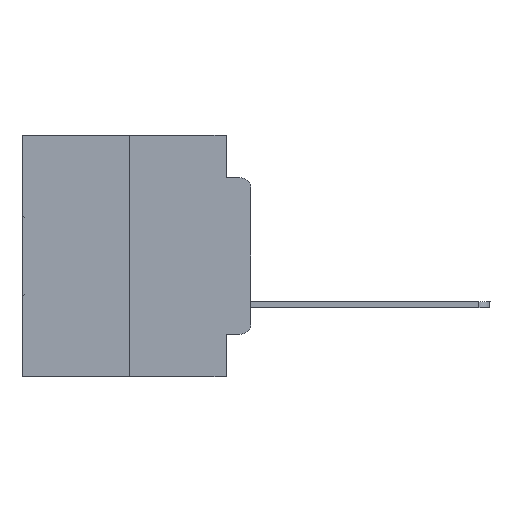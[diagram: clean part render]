
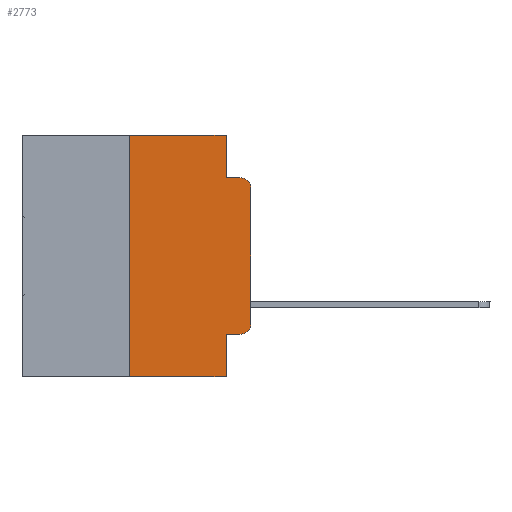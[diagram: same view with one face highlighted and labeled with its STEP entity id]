
A CAD part, left-side view. The second image highlights one B-rep face of the part: STEP entity #2773.
In plain terms, the highlighted planar face has unit normal (-1, 0, 0).
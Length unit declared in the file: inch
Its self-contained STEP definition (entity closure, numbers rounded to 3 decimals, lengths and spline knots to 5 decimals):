
#4 = VERTEX_POINT ( 'NONE', #14316 ) ;
#375 = LINE ( 'NONE', #21339, #31146 ) ;
#378 = CARTESIAN_POINT ( 'NONE',  ( 0., 0.02, -0.0885 ) ) ;
#1081 = VERTEX_POINT ( 'NONE', #2735 ) ;
#2509 = CARTESIAN_POINT ( 'NONE',  ( 0., 0.02, -0.4115 ) ) ;
#2677 = VERTEX_POINT ( 'NONE', #24000 ) ;
#2735 = CARTESIAN_POINT ( 'NONE',  ( 0., 0.051, 0. ) ) ;
#2773 = ADVANCED_FACE ( 'NONE', ( #18692 ), #16845, .F. ) ;
#2887 = CARTESIAN_POINT ( 'NONE',  ( 0., 0., 0. ) ) ;
#3258 = VERTEX_POINT ( 'NONE', #2509 ) ;
#3764 = VECTOR ( 'NONE', #27552, 39.37008 ) ;
#3989 = DIRECTION ( 'NONE',  ( 0., 0., -1. ) ) ;
#4099 = ORIENTED_EDGE ( 'NONE', *, *, #5111, .F. ) ;
#4485 = CARTESIAN_POINT ( 'NONE',  ( 0., 0.051, -0.4115 ) ) ;
#4489 = CARTESIAN_POINT ( 'NONE',  ( 0., 0.051, -0.0885 ) ) ;
#4535 = VERTEX_POINT ( 'NONE', #17187 ) ;
#5091 = CARTESIAN_POINT ( 'NONE',  ( 0., 0.25, 0. ) ) ;
#5111 = EDGE_CURVE ( 'NONE', #12647, #26670, #29083, .T. ) ;
#6140 = CIRCLE ( 'NONE', #15442, 0.02 ) ;
#6686 = CARTESIAN_POINT ( 'NONE',  ( 0., 0.473, -0.5 ) ) ;
#6789 = DIRECTION ( 'NONE',  ( 1., 0., 0. ) ) ;
#6993 = LINE ( 'NONE', #21901, #21143 ) ;
#7224 = VECTOR ( 'NONE', #22726, 39.37008 ) ;
#7760 = ORIENTED_EDGE ( 'NONE', *, *, #19105, .F. ) ;
#8039 = EDGE_CURVE ( 'NONE', #4535, #29188, #31337, .T. ) ;
#8540 = DIRECTION ( 'NONE',  ( 0., -1., 0. ) ) ;
#9163 = DIRECTION ( 'NONE',  ( 0., 0., -1. ) ) ;
#9197 = CARTESIAN_POINT ( 'NONE',  ( 0., 0.02, -0.3915 ) ) ;
#10219 = ORIENTED_EDGE ( 'NONE', *, *, #20925, .T. ) ;
#12647 = VERTEX_POINT ( 'NONE', #20083 ) ;
#12903 = ORIENTED_EDGE ( 'NONE', *, *, #32550, .F. ) ;
#13345 = CARTESIAN_POINT ( 'NONE',  ( 0., 0.051, 0. ) ) ;
#14316 = CARTESIAN_POINT ( 'NONE',  ( 0., 0.051, -0.4115 ) ) ;
#15442 = AXIS2_PLACEMENT_3D ( 'NONE', #9197, #19457, #3989 ) ;
#16789 = ORIENTED_EDGE ( 'NONE', *, *, #24259, .T. ) ;
#16845 = PLANE ( 'NONE',  #33060 ) ;
#16944 = DIRECTION ( 'NONE',  ( 0., 0., -1. ) ) ;
#17187 = CARTESIAN_POINT ( 'NONE',  ( 0., 0.25, -0.5 ) ) ;
#17409 = ORIENTED_EDGE ( 'NONE', *, *, #23856, .T. ) ;
#18180 = EDGE_CURVE ( 'NONE', #4535, #2677, #31624, .T. ) ;
#18672 = LINE ( 'NONE', #13345, #25993 ) ;
#18692 = FACE_OUTER_BOUND ( 'NONE', #29933, .T. ) ;
#19105 = EDGE_CURVE ( 'NONE', #29188, #1081, #375, .T. ) ;
#19259 = DIRECTION ( 'NONE',  ( 0., 0., -1. ) ) ;
#19457 = DIRECTION ( 'NONE',  ( -1., 0., 0. ) ) ;
#19828 = CARTESIAN_POINT ( 'NONE',  ( 0., 0.25, 0. ) ) ;
#20083 = CARTESIAN_POINT ( 'NONE',  ( 0., 0.051, -0.0885 ) ) ;
#20651 = CARTESIAN_POINT ( 'NONE',  ( 0., 0., -0.3915 ) ) ;
#20829 = LINE ( 'NONE', #2887, #23971 ) ;
#20925 = EDGE_CURVE ( 'NONE', #4, #3258, #33416, .T. ) ;
#21143 = VECTOR ( 'NONE', #19259, 39.37008 ) ;
#21339 = CARTESIAN_POINT ( 'NONE',  ( 0., 0.473, 0. ) ) ;
#21424 = VERTEX_POINT ( 'NONE', #25045 ) ;
#21901 = CARTESIAN_POINT ( 'NONE',  ( 0., 0.051, 0. ) ) ;
#22177 = DIRECTION ( 'NONE',  ( -1., 0., 0. ) ) ;
#22306 = CARTESIAN_POINT ( 'NONE',  ( 0., 0.473, 0. ) ) ;
#22324 = CIRCLE ( 'NONE', #25738, 0.02 ) ;
#22488 = DIRECTION ( 'NONE',  ( 0., -1., 0. ) ) ;
#22621 = ORIENTED_EDGE ( 'NONE', *, *, #8039, .F. ) ;
#22726 = DIRECTION ( 'NONE',  ( 0., -1., 0. ) ) ;
#22873 = VERTEX_POINT ( 'NONE', #20651 ) ;
#23856 = EDGE_CURVE ( 'NONE', #21424, #26670, #22324, .T. ) ;
#23971 = VECTOR ( 'NONE', #24060, 39.37008 ) ;
#24000 = CARTESIAN_POINT ( 'NONE',  ( 0., 0.051, -0.5 ) ) ;
#24060 = DIRECTION ( 'NONE',  ( 0., 0., 1. ) ) ;
#24259 = EDGE_CURVE ( 'NONE', #22873, #21424, #20829, .T. ) ;
#25045 = CARTESIAN_POINT ( 'NONE',  ( 0., 0., -0.1085 ) ) ;
#25738 = AXIS2_PLACEMENT_3D ( 'NONE', #30196, #22177, #16944 ) ;
#25819 = ORIENTED_EDGE ( 'NONE', *, *, #32140, .T. ) ;
#25955 = VECTOR ( 'NONE', #32615, 39.37008 ) ;
#25964 = EDGE_CURVE ( 'NONE', #4, #2677, #6993, .T. ) ;
#25993 = VECTOR ( 'NONE', #29517, 39.37008 ) ;
#26670 = VERTEX_POINT ( 'NONE', #378 ) ;
#27552 = DIRECTION ( 'NONE',  ( 0., 0., 1. ) ) ;
#28045 = ORIENTED_EDGE ( 'NONE', *, *, #25964, .F. ) ;
#29083 = LINE ( 'NONE', #4489, #7224 ) ;
#29188 = VERTEX_POINT ( 'NONE', #5091 ) ;
#29517 = DIRECTION ( 'NONE',  ( 0., 0., -1. ) ) ;
#29933 = EDGE_LOOP ( 'NONE', ( #16789, #17409, #4099, #12903, #7760, #22621, #32265, #28045, #10219, #25819 ) ) ;
#30196 = CARTESIAN_POINT ( 'NONE',  ( 0., 0.02, -0.1085 ) ) ;
#31146 = VECTOR ( 'NONE', #8540, 39.37008 ) ;
#31337 = LINE ( 'NONE', #19828, #3764 ) ;
#31624 = LINE ( 'NONE', #6686, #25955 ) ;
#31780 = VECTOR ( 'NONE', #22488, 39.37008 ) ;
#32140 = EDGE_CURVE ( 'NONE', #3258, #22873, #6140, .T. ) ;
#32265 = ORIENTED_EDGE ( 'NONE', *, *, #18180, .T. ) ;
#32550 = EDGE_CURVE ( 'NONE', #1081, #12647, #18672, .T. ) ;
#32615 = DIRECTION ( 'NONE',  ( 0., -1., 0. ) ) ;
#33060 = AXIS2_PLACEMENT_3D ( 'NONE', #22306, #6789, #9163 ) ;
#33416 = LINE ( 'NONE', #4485, #31780 ) ;
